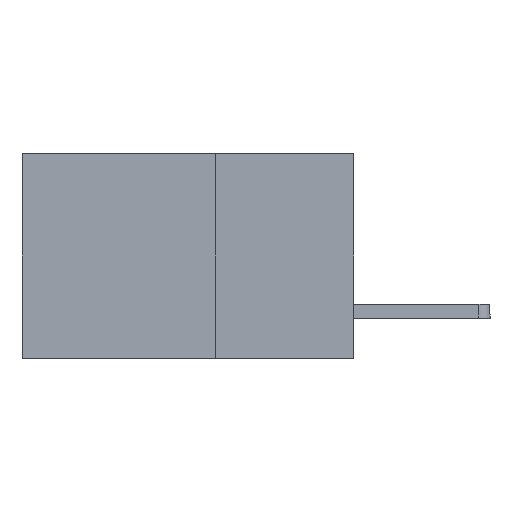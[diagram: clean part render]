
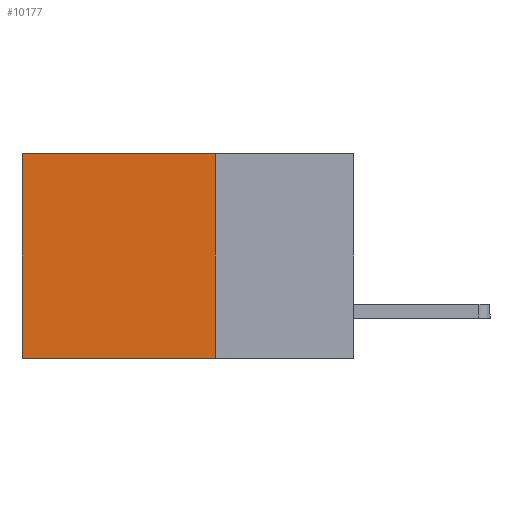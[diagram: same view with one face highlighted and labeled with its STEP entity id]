
A CAD part, left-side view. The second image highlights one B-rep face of the part: STEP entity #10177.
In plain terms, the highlighted planar face has unit normal (-1, 0, 0).
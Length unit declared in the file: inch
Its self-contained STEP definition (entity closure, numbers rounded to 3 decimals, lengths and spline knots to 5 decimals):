
#52 = ORIENTED_EDGE ( 'NONE', *, *, #496, .T. ) ;
#496 = EDGE_CURVE ( 'NONE', #10792, #6896, #10831, .T. ) ;
#537 = DIRECTION ( 'NONE',  ( 1., 0., 0. ) ) ;
#580 = CARTESIAN_POINT ( 'NONE',  ( 0.2875, 0.6, -0.37 ) ) ;
#747 = CARTESIAN_POINT ( 'NONE',  ( 0.2875, 0.25, 0. ) ) ;
#1462 = VERTEX_POINT ( 'NONE', #4538 ) ;
#1498 = FACE_OUTER_BOUND ( 'NONE', #2547, .T. ) ;
#1554 = VECTOR ( 'NONE', #10223, 39.37008 ) ;
#1591 = CARTESIAN_POINT ( 'NONE',  ( 0.2875, 0.6, 0. ) ) ;
#1787 = VECTOR ( 'NONE', #3481, 39.37008 ) ;
#2547 = EDGE_LOOP ( 'NONE', ( #52, #4393, #8369, #8115 ) ) ;
#2719 = CARTESIAN_POINT ( 'NONE',  ( 0.2875, 0.25, -0.37 ) ) ;
#2921 = LINE ( 'NONE', #9321, #5593 ) ;
#3185 = CARTESIAN_POINT ( 'NONE',  ( 0.2875, 0.25, 0. ) ) ;
#3306 = CARTESIAN_POINT ( 'NONE',  ( 0.2875, 0.6, 0. ) ) ;
#3313 = EDGE_CURVE ( 'NONE', #1462, #5864, #2921, .T. ) ;
#3461 = EDGE_CURVE ( 'NONE', #1462, #10792, #3924, .T. ) ;
#3481 = DIRECTION ( 'NONE',  ( 0., 0., -1. ) ) ;
#3924 = LINE ( 'NONE', #747, #1554 ) ;
#4321 = AXIS2_PLACEMENT_3D ( 'NONE', #3185, #537, #6761 ) ;
#4393 = ORIENTED_EDGE ( 'NONE', *, *, #9352, .F. ) ;
#4538 = CARTESIAN_POINT ( 'NONE',  ( 0.2875, 0.25, 0. ) ) ;
#5542 = CARTESIAN_POINT ( 'NONE',  ( 0.2875, 0.25, -0.37 ) ) ;
#5593 = VECTOR ( 'NONE', #8475, 39.37008 ) ;
#5864 = VERTEX_POINT ( 'NONE', #2719 ) ;
#6451 = DIRECTION ( 'NONE',  ( 0., 1., 0. ) ) ;
#6761 = DIRECTION ( 'NONE',  ( 0., 0., -1. ) ) ;
#6896 = VERTEX_POINT ( 'NONE', #580 ) ;
#8115 = ORIENTED_EDGE ( 'NONE', *, *, #3461, .T. ) ;
#8369 = ORIENTED_EDGE ( 'NONE', *, *, #3313, .F. ) ;
#8475 = DIRECTION ( 'NONE',  ( 0., 0., -1. ) ) ;
#9321 = CARTESIAN_POINT ( 'NONE',  ( 0.2875, 0.25, 0. ) ) ;
#9352 = EDGE_CURVE ( 'NONE', #5864, #6896, #10556, .T. ) ;
#9972 = PLANE ( 'NONE',  #4321 ) ;
#10177 = ADVANCED_FACE ( 'NONE', ( #1498 ), #9972, .F. ) ;
#10223 = DIRECTION ( 'NONE',  ( 0., 1., 0. ) ) ;
#10302 = VECTOR ( 'NONE', #6451, 39.37008 ) ;
#10556 = LINE ( 'NONE', #5542, #10302 ) ;
#10792 = VERTEX_POINT ( 'NONE', #1591 ) ;
#10831 = LINE ( 'NONE', #3306, #1787 ) ;
